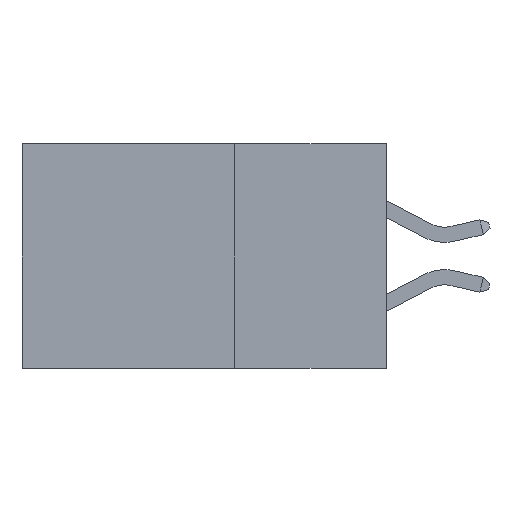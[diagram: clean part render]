
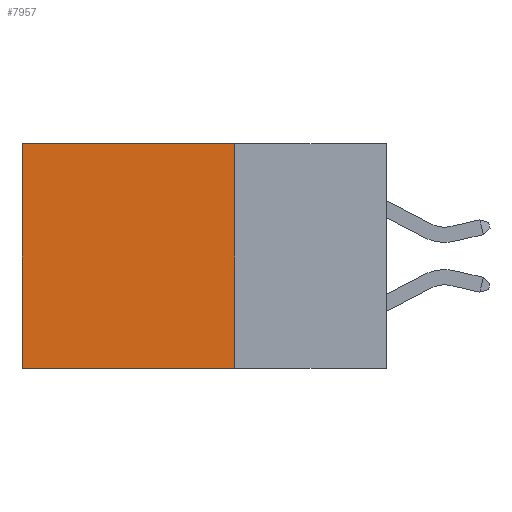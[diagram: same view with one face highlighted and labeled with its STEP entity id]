
A CAD part, left-side view. The second image highlights one B-rep face of the part: STEP entity #7957.
In plain terms, the highlighted planar face has unit normal (-1, 0, 0).
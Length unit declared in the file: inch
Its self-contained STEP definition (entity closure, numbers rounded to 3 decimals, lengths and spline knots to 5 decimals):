
#131 = VECTOR ( 'NONE', #1165, 39.37008 ) ;
#233 = CARTESIAN_POINT ( 'NONE',  ( 0.2615, 0.6, 0. ) ) ;
#248 = VECTOR ( 'NONE', #6871, 39.37008 ) ;
#475 = CARTESIAN_POINT ( 'NONE',  ( 0.2615, 0.25, -0.37 ) ) ;
#585 = EDGE_CURVE ( 'NONE', #3872, #7110, #6034, .T. ) ;
#1021 = EDGE_CURVE ( 'NONE', #3872, #2081, #6767, .T. ) ;
#1165 = DIRECTION ( 'NONE',  ( 0., 0., -1. ) ) ;
#1318 = VECTOR ( 'NONE', #3116, 39.37008 ) ;
#2081 = VERTEX_POINT ( 'NONE', #233 ) ;
#2112 = DIRECTION ( 'NONE',  ( 0., 1., 0. ) ) ;
#2144 = EDGE_CURVE ( 'NONE', #7110, #7636, #5382, .T. ) ;
#3005 = CARTESIAN_POINT ( 'NONE',  ( 0.2615, 0.25, 0. ) ) ;
#3116 = DIRECTION ( 'NONE',  ( 0., 1., 0. ) ) ;
#3147 = ORIENTED_EDGE ( 'NONE', *, *, #1021, .T. ) ;
#3214 = DIRECTION ( 'NONE',  ( 1., 0., 0. ) ) ;
#3523 = VECTOR ( 'NONE', #2112, 39.37008 ) ;
#3872 = VERTEX_POINT ( 'NONE', #3005 ) ;
#4335 = ORIENTED_EDGE ( 'NONE', *, *, #2144, .F. ) ;
#4396 = AXIS2_PLACEMENT_3D ( 'NONE', #475, #3214, #7280 ) ;
#4723 = EDGE_LOOP ( 'NONE', ( #5720, #4335, #7903, #3147 ) ) ;
#4940 = CARTESIAN_POINT ( 'NONE',  ( 0.2615, 0.25, 0. ) ) ;
#5033 = EDGE_CURVE ( 'NONE', #2081, #7636, #7627, .T. ) ;
#5382 = LINE ( 'NONE', #5874, #1318 ) ;
#5720 = ORIENTED_EDGE ( 'NONE', *, *, #5033, .T. ) ;
#5745 = CARTESIAN_POINT ( 'NONE',  ( 0.2615, 0.6, -0.37 ) ) ;
#5874 = CARTESIAN_POINT ( 'NONE',  ( 0.2615, 0.25, -0.37 ) ) ;
#6026 = PLANE ( 'NONE',  #4396 ) ;
#6034 = LINE ( 'NONE', #6598, #131 ) ;
#6598 = CARTESIAN_POINT ( 'NONE',  ( 0.2615, 0.25, -0.37 ) ) ;
#6767 = LINE ( 'NONE', #4940, #3523 ) ;
#6871 = DIRECTION ( 'NONE',  ( 0., 0., -1. ) ) ;
#7110 = VERTEX_POINT ( 'NONE', #8354 ) ;
#7280 = DIRECTION ( 'NONE',  ( 0., 0., -1. ) ) ;
#7627 = LINE ( 'NONE', #5745, #248 ) ;
#7636 = VERTEX_POINT ( 'NONE', #8268 ) ;
#7903 = ORIENTED_EDGE ( 'NONE', *, *, #585, .F. ) ;
#7957 = ADVANCED_FACE ( 'NONE', ( #8625 ), #6026, .F. ) ;
#8268 = CARTESIAN_POINT ( 'NONE',  ( 0.2615, 0.6, -0.37 ) ) ;
#8354 = CARTESIAN_POINT ( 'NONE',  ( 0.2615, 0.25, -0.37 ) ) ;
#8625 = FACE_OUTER_BOUND ( 'NONE', #4723, .T. ) ;
